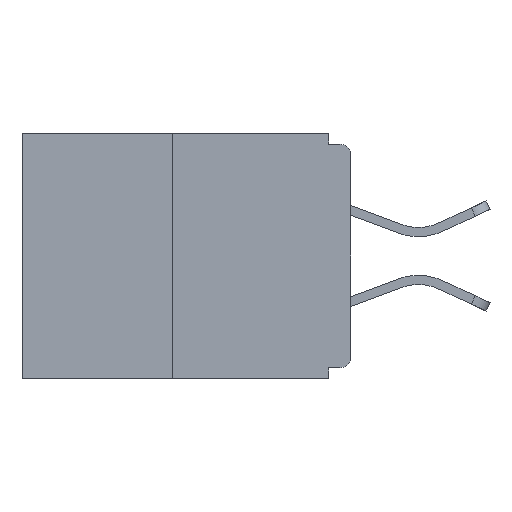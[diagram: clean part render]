
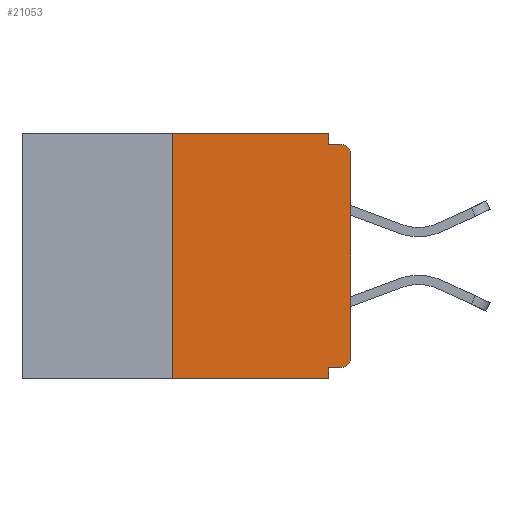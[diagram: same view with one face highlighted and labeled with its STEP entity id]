
A CAD part, left-side view. The second image highlights one B-rep face of the part: STEP entity #21053.
In plain terms, the highlighted planar face has unit normal (-1, 0, 0).
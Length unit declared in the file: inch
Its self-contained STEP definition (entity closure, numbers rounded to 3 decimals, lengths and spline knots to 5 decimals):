
#347 = LINE ( 'NONE', #21976, #6048 ) ;
#1361 = VERTEX_POINT ( 'NONE', #5906 ) ;
#2242 = EDGE_CURVE ( 'NONE', #1361, #20930, #3861, .T. ) ;
#2849 = EDGE_CURVE ( 'NONE', #8632, #21805, #19246, .T. ) ;
#2863 = CARTESIAN_POINT ( 'NONE',  ( 0., 0.031, -0.328 ) ) ;
#3861 = LINE ( 'NONE', #15220, #22464 ) ;
#5523 = CARTESIAN_POINT ( 'NONE',  ( 0., 0.25, -0.343 ) ) ;
#5811 = VECTOR ( 'NONE', #10293, 39.37008 ) ;
#5906 = CARTESIAN_POINT ( 'NONE',  ( 0., 0.25, 0. ) ) ;
#6048 = VECTOR ( 'NONE', #26263, 39.37008 ) ;
#6067 = ORIENTED_EDGE ( 'NONE', *, *, #27246, .F. ) ;
#6511 = CARTESIAN_POINT ( 'NONE',  ( 0., 0.46, 0. ) ) ;
#6721 = CARTESIAN_POINT ( 'NONE',  ( 0., 0., -0.03 ) ) ;
#6791 = VERTEX_POINT ( 'NONE', #10193 ) ;
#6977 = DIRECTION ( 'NONE',  ( 0., 0., -1. ) ) ;
#7559 = LINE ( 'NONE', #21434, #5811 ) ;
#7964 = DIRECTION ( 'NONE',  ( 0., -1., 0. ) ) ;
#8189 = EDGE_CURVE ( 'NONE', #8632, #25487, #347, .T. ) ;
#8550 = CARTESIAN_POINT ( 'NONE',  ( 0., 0., -0.015 ) ) ;
#8632 = VERTEX_POINT ( 'NONE', #20871 ) ;
#9784 = DIRECTION ( 'NONE',  ( 0., 0., 1. ) ) ;
#9828 = CARTESIAN_POINT ( 'NONE',  ( 0., 0.031, -0.343 ) ) ;
#10095 = EDGE_CURVE ( 'NONE', #24389, #1361, #15233, .T. ) ;
#10193 = CARTESIAN_POINT ( 'NONE',  ( 0., 0.031, -0.343 ) ) ;
#10293 = DIRECTION ( 'NONE',  ( 0., 0., 1. ) ) ;
#10553 = ORIENTED_EDGE ( 'NONE', *, *, #2242, .F. ) ;
#10635 = EDGE_CURVE ( 'NONE', #20930, #14707, #12715, .T. ) ;
#10709 = DIRECTION ( 'NONE',  ( 0., -1., 0. ) ) ;
#10860 = CARTESIAN_POINT ( 'NONE',  ( 0., 0.031, -0.015 ) ) ;
#11413 = CARTESIAN_POINT ( 'NONE',  ( 0., 0.015, -0.313 ) ) ;
#11484 = EDGE_CURVE ( 'NONE', #25487, #6791, #23814, .T. ) ;
#12715 = LINE ( 'NONE', #16513, #26995 ) ;
#12977 = ORIENTED_EDGE ( 'NONE', *, *, #20900, .T. ) ;
#13606 = EDGE_CURVE ( 'NONE', #21805, #27319, #7559, .T. ) ;
#13708 = VECTOR ( 'NONE', #7964, 39.37008 ) ;
#13795 = VECTOR ( 'NONE', #9784, 39.37008 ) ;
#14344 = CARTESIAN_POINT ( 'NONE',  ( 0., 0.031, 0. ) ) ;
#14449 = DIRECTION ( 'NONE',  ( 0., 0., -1. ) ) ;
#14707 = VERTEX_POINT ( 'NONE', #10860 ) ;
#15220 = CARTESIAN_POINT ( 'NONE',  ( 0., 0.46, 0. ) ) ;
#15233 = LINE ( 'NONE', #23794, #13795 ) ;
#15471 = AXIS2_PLACEMENT_3D ( 'NONE', #11413, #24818, #18051 ) ;
#15724 = AXIS2_PLACEMENT_3D ( 'NONE', #25839, #28128, #14449 ) ;
#15774 = ORIENTED_EDGE ( 'NONE', *, *, #28292, .T. ) ;
#15840 = LINE ( 'NONE', #28853, #13708 ) ;
#16513 = CARTESIAN_POINT ( 'NONE',  ( 0., 0.031, 0. ) ) ;
#16648 = LINE ( 'NONE', #8550, #22018 ) ;
#16705 = CARTESIAN_POINT ( 'NONE',  ( 0., 0.015, -0.015 ) ) ;
#18024 = ORIENTED_EDGE ( 'NONE', *, *, #8189, .F. ) ;
#18051 = DIRECTION ( 'NONE',  ( 0., 0., -1. ) ) ;
#18252 = AXIS2_PLACEMENT_3D ( 'NONE', #6511, #20357, #27024 ) ;
#18667 = DIRECTION ( 'NONE',  ( 0., -1., 0. ) ) ;
#19083 = FACE_OUTER_BOUND ( 'NONE', #24914, .T. ) ;
#19231 = ORIENTED_EDGE ( 'NONE', *, *, #13606, .T. ) ;
#19246 = CIRCLE ( 'NONE', #15471, 0.015 ) ;
#20279 = VERTEX_POINT ( 'NONE', #16705 ) ;
#20357 = DIRECTION ( 'NONE',  ( 1., 0., 0. ) ) ;
#20790 = ORIENTED_EDGE ( 'NONE', *, *, #11484, .F. ) ;
#20871 = CARTESIAN_POINT ( 'NONE',  ( 0., 0.015, -0.328 ) ) ;
#20900 = EDGE_CURVE ( 'NONE', #27319, #20279, #24083, .T. ) ;
#20930 = VERTEX_POINT ( 'NONE', #14344 ) ;
#21053 = ADVANCED_FACE ( 'NONE', ( #19083 ), #25119, .F. ) ;
#21434 = CARTESIAN_POINT ( 'NONE',  ( 0., 0., 0. ) ) ;
#21805 = VERTEX_POINT ( 'NONE', #25673 ) ;
#21813 = ORIENTED_EDGE ( 'NONE', *, *, #10095, .F. ) ;
#21976 = CARTESIAN_POINT ( 'NONE',  ( 0., 0., -0.328 ) ) ;
#22018 = VECTOR ( 'NONE', #18667, 39.37008 ) ;
#22464 = VECTOR ( 'NONE', #10709, 39.37008 ) ;
#23794 = CARTESIAN_POINT ( 'NONE',  ( 0., 0.25, 0. ) ) ;
#23814 = LINE ( 'NONE', #9828, #26309 ) ;
#24083 = CIRCLE ( 'NONE', #15724, 0.015 ) ;
#24389 = VERTEX_POINT ( 'NONE', #5523 ) ;
#24818 = DIRECTION ( 'NONE',  ( -1., 0., 0. ) ) ;
#24914 = EDGE_LOOP ( 'NONE', ( #10553, #21813, #15774, #20790, #18024, #26880, #19231, #12977, #6067, #28857 ) ) ;
#25119 = PLANE ( 'NONE',  #18252 ) ;
#25487 = VERTEX_POINT ( 'NONE', #2863 ) ;
#25673 = CARTESIAN_POINT ( 'NONE',  ( 0., 0., -0.313 ) ) ;
#25839 = CARTESIAN_POINT ( 'NONE',  ( 0., 0.015, -0.03 ) ) ;
#26263 = DIRECTION ( 'NONE',  ( 0., 1., 0. ) ) ;
#26309 = VECTOR ( 'NONE', #28001, 39.37008 ) ;
#26880 = ORIENTED_EDGE ( 'NONE', *, *, #2849, .T. ) ;
#26995 = VECTOR ( 'NONE', #6977, 39.37008 ) ;
#27024 = DIRECTION ( 'NONE',  ( 0., 0., -1. ) ) ;
#27246 = EDGE_CURVE ( 'NONE', #14707, #20279, #16648, .T. ) ;
#27319 = VERTEX_POINT ( 'NONE', #6721 ) ;
#28001 = DIRECTION ( 'NONE',  ( 0., 0., -1. ) ) ;
#28128 = DIRECTION ( 'NONE',  ( -1., 0., 0. ) ) ;
#28292 = EDGE_CURVE ( 'NONE', #24389, #6791, #15840, .T. ) ;
#28853 = CARTESIAN_POINT ( 'NONE',  ( 0., 0.46, -0.343 ) ) ;
#28857 = ORIENTED_EDGE ( 'NONE', *, *, #10635, .F. ) ;
